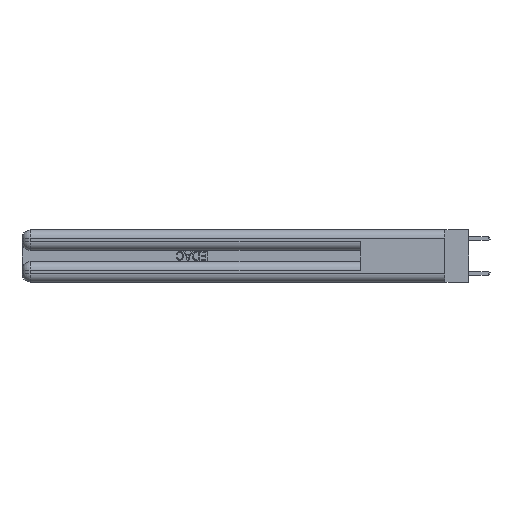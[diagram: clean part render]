
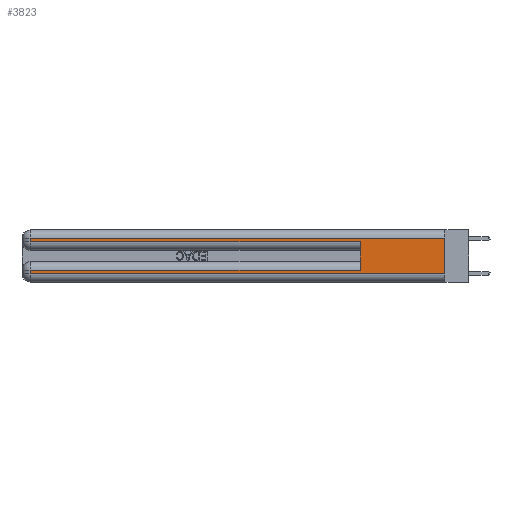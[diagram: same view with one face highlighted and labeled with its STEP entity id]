
A CAD part, left-side view. The second image highlights one B-rep face of the part: STEP entity #3823.
In plain terms, the highlighted planar face has unit normal (-1, 0, 0).
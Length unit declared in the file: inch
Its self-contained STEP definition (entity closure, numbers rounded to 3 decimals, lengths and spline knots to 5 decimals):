
#232 = CARTESIAN_POINT ( 'NONE',  ( 0., 2.94, 0.285 ) ) ;
#713 = CARTESIAN_POINT ( 'NONE',  ( 0., 2.94, 0.37 ) ) ;
#1232 = VERTEX_POINT ( 'NONE', #12662 ) ;
#2326 = CARTESIAN_POINT ( 'NONE',  ( 0., 2.94, 0.06 ) ) ;
#2327 = DIRECTION ( 'NONE',  ( 0., 0., -1. ) ) ;
#2675 = LINE ( 'NONE', #8201, #29676 ) ;
#3029 = LINE ( 'NONE', #5542, #26176 ) ;
#3202 = ORIENTED_EDGE ( 'NONE', *, *, #10332, .T. ) ;
#3579 = ORIENTED_EDGE ( 'NONE', *, *, #16070, .F. ) ;
#3823 = ADVANCED_FACE ( 'NONE', ( #34339 ), #15209, .F. ) ;
#4022 = EDGE_CURVE ( 'NONE', #1232, #14078, #3029, .T. ) ;
#4213 = CARTESIAN_POINT ( 'NONE',  ( 0., 0.6, 0.085 ) ) ;
#5284 = VERTEX_POINT ( 'NONE', #2326 ) ;
#5542 = CARTESIAN_POINT ( 'NONE',  ( 0., 0., 0.31 ) ) ;
#5901 = EDGE_CURVE ( 'NONE', #24317, #6765, #17171, .T. ) ;
#6607 = LINE ( 'NONE', #31892, #31018 ) ;
#6732 = CARTESIAN_POINT ( 'NONE',  ( 0., 0., 0.06 ) ) ;
#6765 = VERTEX_POINT ( 'NONE', #13206 ) ;
#8058 = DIRECTION ( 'NONE',  ( 0., 0., -1. ) ) ;
#8201 = CARTESIAN_POINT ( 'NONE',  ( 0., 2.94, 0.37 ) ) ;
#8364 = CARTESIAN_POINT ( 'NONE',  ( 0., 0., 0.06 ) ) ;
#8789 = EDGE_CURVE ( 'NONE', #15952, #5284, #25161, .T. ) ;
#9073 = EDGE_CURVE ( 'NONE', #25739, #15952, #16689, .T. ) ;
#9910 = VECTOR ( 'NONE', #8058, 39.37008 ) ;
#10332 = EDGE_CURVE ( 'NONE', #14078, #24317, #2675, .T. ) ;
#10526 = DIRECTION ( 'NONE',  ( 1., 0., 0. ) ) ;
#10874 = DIRECTION ( 'NONE',  ( 0., 0., -1. ) ) ;
#11348 = DIRECTION ( 'NONE',  ( 0., 1., 0. ) ) ;
#11599 = DIRECTION ( 'NONE',  ( 0., 0., -1. ) ) ;
#12662 = CARTESIAN_POINT ( 'NONE',  ( 0., 0., 0.31 ) ) ;
#13071 = AXIS2_PLACEMENT_3D ( 'NONE', #16040, #10526, #2327 ) ;
#13093 = VECTOR ( 'NONE', #11348, 39.37008 ) ;
#13206 = CARTESIAN_POINT ( 'NONE',  ( 0., 0.6, 0.285 ) ) ;
#14078 = VERTEX_POINT ( 'NONE', #21938 ) ;
#15209 = PLANE ( 'NONE',  #13071 ) ;
#15806 = EDGE_CURVE ( 'NONE', #1232, #25093, #26258, .T. ) ;
#15952 = VERTEX_POINT ( 'NONE', #19282 ) ;
#16040 = CARTESIAN_POINT ( 'NONE',  ( 0., 0., 0.37 ) ) ;
#16070 = EDGE_CURVE ( 'NONE', #25739, #6765, #6607, .T. ) ;
#16689 = LINE ( 'NONE', #27586, #13093 ) ;
#17047 = VECTOR ( 'NONE', #25404, 39.37008 ) ;
#17171 = LINE ( 'NONE', #20037, #17047 ) ;
#19244 = DIRECTION ( 'NONE',  ( 0., -1., 0. ) ) ;
#19282 = CARTESIAN_POINT ( 'NONE',  ( 0., 2.94, 0.085 ) ) ;
#20037 = CARTESIAN_POINT ( 'NONE',  ( 0., 0., 0.285 ) ) ;
#20987 = DIRECTION ( 'NONE',  ( 0., 0., 1. ) ) ;
#21549 = VECTOR ( 'NONE', #19244, 39.37008 ) ;
#21938 = CARTESIAN_POINT ( 'NONE',  ( 0., 2.94, 0.31 ) ) ;
#22089 = ORIENTED_EDGE ( 'NONE', *, *, #5901, .T. ) ;
#22168 = VECTOR ( 'NONE', #11599, 39.37008 ) ;
#24207 = EDGE_LOOP ( 'NONE', ( #25157, #29813, #3202, #22089, #3579, #31187, #24351, #32564 ) ) ;
#24317 = VERTEX_POINT ( 'NONE', #232 ) ;
#24351 = ORIENTED_EDGE ( 'NONE', *, *, #8789, .T. ) ;
#25093 = VERTEX_POINT ( 'NONE', #6732 ) ;
#25157 = ORIENTED_EDGE ( 'NONE', *, *, #15806, .F. ) ;
#25161 = LINE ( 'NONE', #713, #22168 ) ;
#25404 = DIRECTION ( 'NONE',  ( 0., -1., 0. ) ) ;
#25739 = VERTEX_POINT ( 'NONE', #4213 ) ;
#26176 = VECTOR ( 'NONE', #27284, 39.37008 ) ;
#26258 = LINE ( 'NONE', #32503, #9910 ) ;
#27284 = DIRECTION ( 'NONE',  ( 0., 1., 0. ) ) ;
#27586 = CARTESIAN_POINT ( 'NONE',  ( 0., 0., 0.085 ) ) ;
#29676 = VECTOR ( 'NONE', #10874, 39.37008 ) ;
#29813 = ORIENTED_EDGE ( 'NONE', *, *, #4022, .T. ) ;
#30992 = EDGE_CURVE ( 'NONE', #5284, #25093, #32813, .T. ) ;
#31018 = VECTOR ( 'NONE', #20987, 39.37008 ) ;
#31187 = ORIENTED_EDGE ( 'NONE', *, *, #9073, .T. ) ;
#31892 = CARTESIAN_POINT ( 'NONE',  ( 0., 0.6, 0.145 ) ) ;
#32503 = CARTESIAN_POINT ( 'NONE',  ( 0., 0., 0.37 ) ) ;
#32564 = ORIENTED_EDGE ( 'NONE', *, *, #30992, .T. ) ;
#32813 = LINE ( 'NONE', #8364, #21549 ) ;
#34339 = FACE_OUTER_BOUND ( 'NONE', #24207, .T. ) ;
